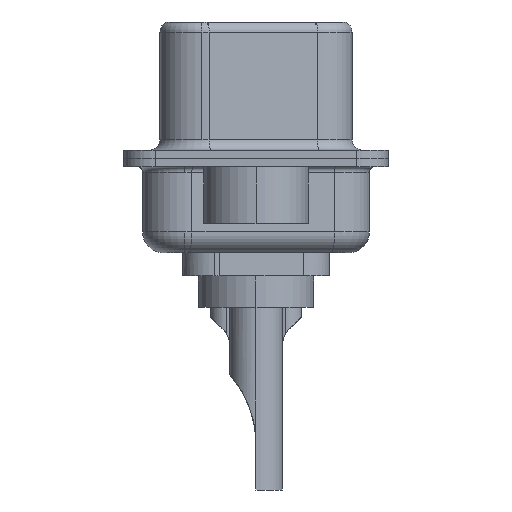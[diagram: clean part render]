
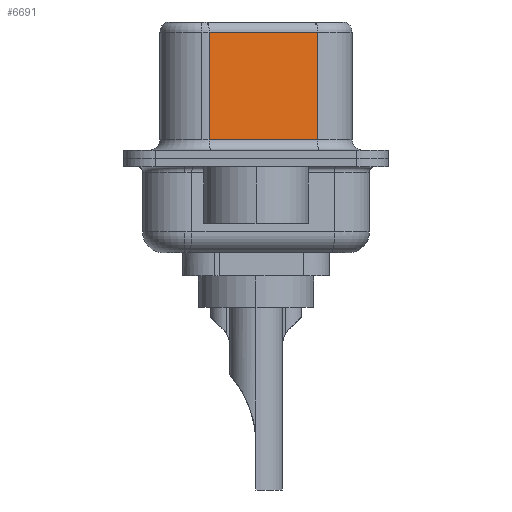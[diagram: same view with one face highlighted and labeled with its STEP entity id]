
A CAD part, left-side view. The second image highlights one B-rep face of the part: STEP entity #6691.
In plain terms, the highlighted planar face has unit normal (-0.985, -0.174, 0).
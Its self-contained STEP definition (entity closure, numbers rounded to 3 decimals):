
#395 = ORIENTED_EDGE ( 'NONE', *, *, #1693, .T. ) ;
#461 = VERTEX_POINT ( 'NONE', #15894 ) ;
#619 = DIRECTION ( 'NONE',  ( 0.985, 0.174, 0. ) ) ;
#1693 = EDGE_CURVE ( 'NONE', #461, #20263, #20968, .T. ) ;
#2301 = FACE_OUTER_BOUND ( 'NONE', #5132, .T. ) ;
#5132 = EDGE_LOOP ( 'NONE', ( #13238, #11596, #395, #18881 ) ) ;
#6169 = AXIS2_PLACEMENT_3D ( 'NONE', #18628, #619, #20022 ) ;
#6353 = LINE ( 'NONE', #18949, #14364 ) ;
#6691 = ADVANCED_FACE ( 'NONE', ( #2301 ), #9226, .F. ) ;
#7276 = VECTOR ( 'NONE', #19405, 1000. ) ;
#8717 = EDGE_CURVE ( 'NONE', #17438, #17761, #22121, .T. ) ;
#8724 = DIRECTION ( 'NONE',  ( 0., 0., -1. ) ) ;
#9226 = PLANE ( 'NONE',  #6169 ) ;
#9371 = CARTESIAN_POINT ( 'NONE',  ( 4.58, -2.927, 0.9 ) ) ;
#9392 = CARTESIAN_POINT ( 'NONE',  ( 4.58, -2.927, 0.9 ) ) ;
#10349 = CARTESIAN_POINT ( 'NONE',  ( 4.58, -2.927, 6.02 ) ) ;
#11456 = EDGE_CURVE ( 'NONE', #20263, #17761, #17883, .T. ) ;
#11596 = ORIENTED_EDGE ( 'NONE', *, *, #13038, .T. ) ;
#13038 = EDGE_CURVE ( 'NONE', #17438, #461, #6353, .T. ) ;
#13238 = ORIENTED_EDGE ( 'NONE', *, *, #8717, .F. ) ;
#13696 = CARTESIAN_POINT ( 'NONE',  ( 3.67, 2.233, 0.9 ) ) ;
#14364 = VECTOR ( 'NONE', #15526, 1000. ) ;
#15526 = DIRECTION ( 'NONE',  ( -0.174, 0.985, 0. ) ) ;
#15894 = CARTESIAN_POINT ( 'NONE',  ( 3.67, 2.233, 6.02 ) ) ;
#16903 = CARTESIAN_POINT ( 'NONE',  ( 4.58, -2.927, 6.52 ) ) ;
#17438 = VERTEX_POINT ( 'NONE', #10349 ) ;
#17761 = VERTEX_POINT ( 'NONE', #9371 ) ;
#17883 = LINE ( 'NONE', #9392, #22004 ) ;
#18628 = CARTESIAN_POINT ( 'NONE',  ( 4.58, -2.927, 6.52 ) ) ;
#18881 = ORIENTED_EDGE ( 'NONE', *, *, #11456, .T. ) ;
#18949 = CARTESIAN_POINT ( 'NONE',  ( 4.58, -2.927, 6.02 ) ) ;
#19405 = DIRECTION ( 'NONE',  ( 0., 0., -1. ) ) ;
#19488 = CARTESIAN_POINT ( 'NONE',  ( 3.67, 2.233, 6.52 ) ) ;
#19683 = DIRECTION ( 'NONE',  ( 0.174, -0.985, 0. ) ) ;
#20022 = DIRECTION ( 'NONE',  ( -0.174, 0.985, 0. ) ) ;
#20263 = VERTEX_POINT ( 'NONE', #13696 ) ;
#20968 = LINE ( 'NONE', #19488, #7276 ) ;
#21552 = VECTOR ( 'NONE', #8724, 1000. ) ;
#22004 = VECTOR ( 'NONE', #19683, 1000. ) ;
#22121 = LINE ( 'NONE', #16903, #21552 ) ;
